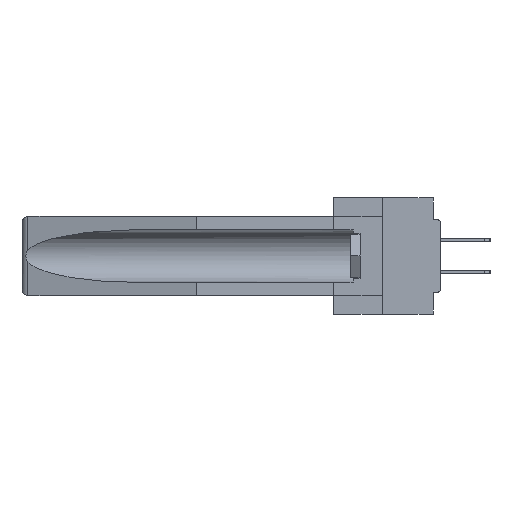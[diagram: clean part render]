
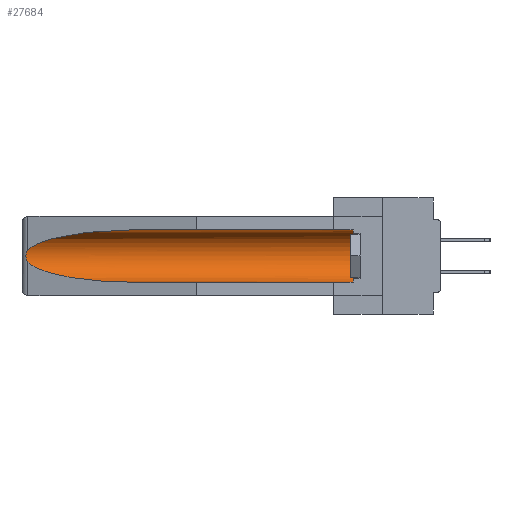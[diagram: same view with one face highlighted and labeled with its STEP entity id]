
A CAD part, left-side view. The second image highlights one B-rep face of the part: STEP entity #27684.
In plain terms, the highlighted cylindrical face has radius 2.857 mm (diameter 5.715 mm), a partial arc.
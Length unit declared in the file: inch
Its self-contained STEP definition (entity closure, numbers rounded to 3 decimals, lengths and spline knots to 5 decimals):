
#587 = CIRCLE ( 'NONE', #2768, 0.1125 ) ;
#622 = CARTESIAN_POINT ( 'NONE',  ( 0.26537, 1.52718, -0.14972 ) ) ;
#641 = ORIENTED_EDGE ( 'NONE', *, *, #20101, .T. ) ;
#994 = CARTESIAN_POINT ( 'NONE',  ( 0.26597, 1.5296, -0.19026 ) ) ;
#1728 = VERTEX_POINT ( 'NONE', #34492 ) ;
#2066 =( BOUNDED_CURVE ( )  B_SPLINE_CURVE ( 3, ( #10273, #7091, #8010, #13327 ),
 .UNSPECIFIED., .F., .F. ) 
 B_SPLINE_CURVE_WITH_KNOTS ( ( 4, 4 ),
 ( 0.1948, 1.5708 ),
 .UNSPECIFIED. ) 
 CURVE ( )  GEOMETRIC_REPRESENTATION_ITEM ( )  RATIONAL_B_SPLINE_CURVE ( ( 1., 0.848, 0.848, 1. ) ) 
 REPRESENTATION_ITEM ( '' )  );
#2768 = AXIS2_PLACEMENT_3D ( 'NONE', #26324, #7105, #31459 ) ;
#6414 = CARTESIAN_POINT ( 'NONE',  ( 0.25451, 1.48313, -0.09465 ) ) ;
#6538 = CARTESIAN_POINT ( 'NONE',  ( 0.26537, 1.52718, -0.14972 ) ) ;
#6546 = CARTESIAN_POINT ( 'NONE',  ( 0.26537, 1.52718, -0.19328 ) ) ;
#7021 = DIRECTION ( 'NONE',  ( 0., 1., 0. ) ) ;
#7091 = CARTESIAN_POINT ( 'NONE',  ( 0.25451, 1.48313, -0.24835 ) ) ;
#7105 = DIRECTION ( 'NONE',  ( 0., -1., 0. ) ) ;
#8010 = CARTESIAN_POINT ( 'NONE',  ( 0.21114, 1.30732, -0.284 ) ) ;
#8096 = AXIS2_PLACEMENT_3D ( 'NONE', #27218, #11050, #27330 ) ;
#8824 = VECTOR ( 'NONE', #7021, 39.37008 ) ;
#9267 = CARTESIAN_POINT ( 'NONE',  ( 0.155, 0.126, -0.059 ) ) ;
#9506 = CARTESIAN_POINT ( 'NONE',  ( 0.155, -0.30754, -0.059 ) ) ;
#10273 = CARTESIAN_POINT ( 'NONE',  ( 0.26537, 1.52718, -0.19328 ) ) ;
#11050 = DIRECTION ( 'NONE',  ( 0., 1., 0. ) ) ;
#11629 = CARTESIAN_POINT ( 'NONE',  ( 0.2675, 1.53308, -0.16763 ) ) ;
#12115 = VERTEX_POINT ( 'NONE', #6538 ) ;
#12855 = EDGE_CURVE ( 'NONE', #34075, #17392, #587, .T. ) ;
#12871 = CARTESIAN_POINT ( 'NONE',  ( 0.155, 0.126, -0.284 ) ) ;
#13327 = CARTESIAN_POINT ( 'NONE',  ( 0.155, 1.07973, -0.284 ) ) ;
#14035 = B_SPLINE_CURVE_WITH_KNOTS ( 'NONE', 3,
 ( #14589, #25262, #30768, #27779, #11629, #28035, #22430, #17343, #994, #6546 ),
 .UNSPECIFIED., .F., .F.,
 ( 4, 2, 2, 2, 4 ),
 ( 0., 0.00029, 0.00058, 0.00087, 0.00117 ),
 .UNSPECIFIED. ) ;
#14589 = CARTESIAN_POINT ( 'NONE',  ( 0.26537, 1.52718, -0.14972 ) ) ;
#14855 = EDGE_CURVE ( 'NONE', #12115, #20368, #14035, .T. ) ;
#16227 =( BOUNDED_CURVE ( )  B_SPLINE_CURVE ( 3, ( #22414, #22664, #6414, #622 ),
 .UNSPECIFIED., .F., .F. ) 
 B_SPLINE_CURVE_WITH_KNOTS ( ( 4, 4 ),
 ( 4.71239, 6.08839 ),
 .UNSPECIFIED. ) 
 CURVE ( )  GEOMETRIC_REPRESENTATION_ITEM ( )  RATIONAL_B_SPLINE_CURVE ( ( 1., 0.848, 0.848, 1. ) ) 
 REPRESENTATION_ITEM ( '' )  );
#16881 = LINE ( 'NONE', #9506, #8824 ) ;
#17343 = CARTESIAN_POINT ( 'NONE',  ( 0.26655, 1.53094, -0.18657 ) ) ;
#17392 = VERTEX_POINT ( 'NONE', #9267 ) ;
#18929 = LINE ( 'NONE', #34857, #21890 ) ;
#20101 = EDGE_CURVE ( 'NONE', #1728, #12115, #16227, .T. ) ;
#20247 = EDGE_CURVE ( 'NONE', #17392, #1728, #16881, .T. ) ;
#20368 = VERTEX_POINT ( 'NONE', #20866 ) ;
#20866 = CARTESIAN_POINT ( 'NONE',  ( 0.26537, 1.52718, -0.19328 ) ) ;
#21890 = VECTOR ( 'NONE', #26586, 39.37008 ) ;
#22172 = FACE_OUTER_BOUND ( 'NONE', #24628, .T. ) ;
#22414 = CARTESIAN_POINT ( 'NONE',  ( 0.155, 1.07973, -0.059 ) ) ;
#22430 = CARTESIAN_POINT ( 'NONE',  ( 0.2673, 1.53269, -0.17917 ) ) ;
#22664 = CARTESIAN_POINT ( 'NONE',  ( 0.21114, 1.30732, -0.059 ) ) ;
#24628 = EDGE_LOOP ( 'NONE', ( #641, #30038, #34799, #32200, #32700, #25402 ) ) ;
#24713 = EDGE_CURVE ( 'NONE', #20368, #24743, #2066, .T. ) ;
#24743 = VERTEX_POINT ( 'NONE', #35130 ) ;
#25262 = CARTESIAN_POINT ( 'NONE',  ( 0.26597, 1.52961, -0.15275 ) ) ;
#25402 = ORIENTED_EDGE ( 'NONE', *, *, #20247, .T. ) ;
#26324 = CARTESIAN_POINT ( 'NONE',  ( 0.155, 0.126, -0.1715 ) ) ;
#26586 = DIRECTION ( 'NONE',  ( 0., 1., 0. ) ) ;
#27218 = CARTESIAN_POINT ( 'NONE',  ( 0.155, -0.30754, -0.1715 ) ) ;
#27330 = DIRECTION ( 'NONE',  ( 0., 0., 1. ) ) ;
#27684 = ADVANCED_FACE ( 'NONE', ( #22172 ), #27706, .F. ) ;
#27706 = CYLINDRICAL_SURFACE ( 'NONE', #8096, 0.1125 ) ;
#27779 = CARTESIAN_POINT ( 'NONE',  ( 0.2673, 1.5327, -0.16383 ) ) ;
#28035 = CARTESIAN_POINT ( 'NONE',  ( 0.2675, 1.53308, -0.17534 ) ) ;
#30038 = ORIENTED_EDGE ( 'NONE', *, *, #14855, .T. ) ;
#30768 = CARTESIAN_POINT ( 'NONE',  ( 0.26654, 1.53092, -0.15636 ) ) ;
#31459 = DIRECTION ( 'NONE',  ( 0., 0., 1. ) ) ;
#32200 = ORIENTED_EDGE ( 'NONE', *, *, #32524, .F. ) ;
#32524 = EDGE_CURVE ( 'NONE', #34075, #24743, #18929, .T. ) ;
#32700 = ORIENTED_EDGE ( 'NONE', *, *, #12855, .T. ) ;
#34075 = VERTEX_POINT ( 'NONE', #12871 ) ;
#34492 = CARTESIAN_POINT ( 'NONE',  ( 0.155, 1.07973, -0.059 ) ) ;
#34799 = ORIENTED_EDGE ( 'NONE', *, *, #24713, .T. ) ;
#34857 = CARTESIAN_POINT ( 'NONE',  ( 0.155, -0.30754, -0.284 ) ) ;
#35130 = CARTESIAN_POINT ( 'NONE',  ( 0.155, 1.07973, -0.284 ) ) ;
